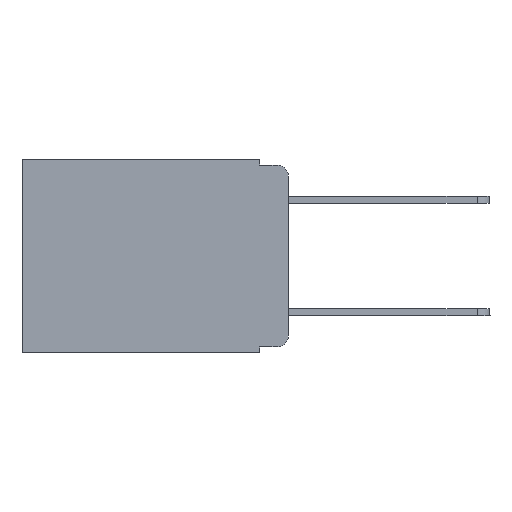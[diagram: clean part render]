
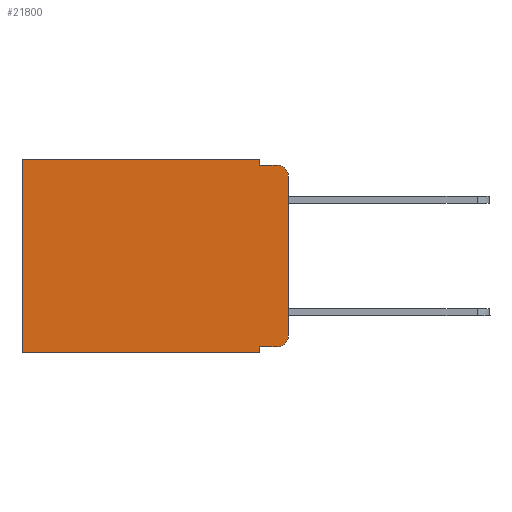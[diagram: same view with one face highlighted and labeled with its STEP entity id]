
A CAD part, left-side view. The second image highlights one B-rep face of the part: STEP entity #21800.
In plain terms, the highlighted planar face has unit normal (-1, 0, 0).
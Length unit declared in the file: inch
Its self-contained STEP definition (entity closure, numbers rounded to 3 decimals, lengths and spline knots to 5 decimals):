
#86 = CARTESIAN_POINT ( 'NONE',  ( 0.298, 0.02, -0.313 ) ) ;
#450 = LINE ( 'NONE', #5903, #1429 ) ;
#1293 = VERTEX_POINT ( 'NONE', #16884 ) ;
#1310 = AXIS2_PLACEMENT_3D ( 'NONE', #14751, #13029, #9602 ) ;
#1429 = VECTOR ( 'NONE', #9416, 39.37008 ) ;
#1767 = ORIENTED_EDGE ( 'NONE', *, *, #3420, .F. ) ;
#1849 = LINE ( 'NONE', #11977, #4859 ) ;
#1903 = LINE ( 'NONE', #16035, #11825 ) ;
#1905 = VERTEX_POINT ( 'NONE', #15480 ) ;
#1956 = LINE ( 'NONE', #10154, #2251 ) ;
#2020 = DIRECTION ( 'NONE',  ( 0., 1., 0. ) ) ;
#2251 = VECTOR ( 'NONE', #13693, 39.37008 ) ;
#2259 = CARTESIAN_POINT ( 'NONE',  ( 0.298, 0., 0. ) ) ;
#2444 = PLANE ( 'NONE',  #1310 ) ;
#2645 = CARTESIAN_POINT ( 'NONE',  ( 0.298, 0., -0.03 ) ) ;
#3133 = DIRECTION ( 'NONE',  ( -1., 0., 0. ) ) ;
#3240 = CARTESIAN_POINT ( 'NONE',  ( 0.298, 0.02, -0.03 ) ) ;
#3420 = EDGE_CURVE ( 'NONE', #14799, #14709, #450, .T. ) ;
#3425 = VECTOR ( 'NONE', #17264, 39.37008 ) ;
#3519 = ORIENTED_EDGE ( 'NONE', *, *, #6052, .F. ) ;
#3616 = DIRECTION ( 'NONE',  ( 0., 0., -1. ) ) ;
#3720 = LINE ( 'NONE', #17625, #22024 ) ;
#3855 = ORIENTED_EDGE ( 'NONE', *, *, #17198, .F. ) ;
#4002 = CARTESIAN_POINT ( 'NONE',  ( 0.298, 0.051, 0. ) ) ;
#4642 = ORIENTED_EDGE ( 'NONE', *, *, #21262, .T. ) ;
#4833 = LINE ( 'NONE', #11771, #11572 ) ;
#4859 = VECTOR ( 'NONE', #8779, 39.37008 ) ;
#4946 = CARTESIAN_POINT ( 'NONE',  ( 0.298, 0.051, -0.01 ) ) ;
#5140 = CIRCLE ( 'NONE', #13151, 0.02 ) ;
#5903 = CARTESIAN_POINT ( 'NONE',  ( 0.298, 0.051, -0.01 ) ) ;
#6052 = EDGE_CURVE ( 'NONE', #12083, #8271, #4833, .T. ) ;
#6919 = DIRECTION ( 'NONE',  ( -1., 0., 0. ) ) ;
#7615 = CARTESIAN_POINT ( 'NONE',  ( 0.298, 0., -0.313 ) ) ;
#8271 = VERTEX_POINT ( 'NONE', #7615 ) ;
#8779 = DIRECTION ( 'NONE',  ( 0., 0., -1. ) ) ;
#8881 = EDGE_CURVE ( 'NONE', #12083, #14709, #5140, .T. ) ;
#9191 = DIRECTION ( 'NONE',  ( 0., 1., 0. ) ) ;
#9244 = VERTEX_POINT ( 'NONE', #14511 ) ;
#9416 = DIRECTION ( 'NONE',  ( 0., -1., 0. ) ) ;
#9452 = EDGE_CURVE ( 'NONE', #16972, #13044, #1956, .T. ) ;
#9602 = DIRECTION ( 'NONE',  ( 0., 0., -1. ) ) ;
#10065 = DIRECTION ( 'NONE',  ( 0., 0., -1. ) ) ;
#10154 = CARTESIAN_POINT ( 'NONE',  ( 0.298, 0.051, -0.333 ) ) ;
#11303 = FACE_OUTER_BOUND ( 'NONE', #18329, .T. ) ;
#11572 = VECTOR ( 'NONE', #18724, 39.37008 ) ;
#11734 = VECTOR ( 'NONE', #9191, 39.37008 ) ;
#11771 = CARTESIAN_POINT ( 'NONE',  ( 0.298, 0., 0. ) ) ;
#11825 = VECTOR ( 'NONE', #3616, 39.37008 ) ;
#11977 = CARTESIAN_POINT ( 'NONE',  ( 0.298, 0.051, 0. ) ) ;
#12024 = CARTESIAN_POINT ( 'NONE',  ( 0.298, 0.051, -0.333 ) ) ;
#12083 = VERTEX_POINT ( 'NONE', #2645 ) ;
#12265 = DIRECTION ( 'NONE',  ( 0., 0., -1. ) ) ;
#12650 = EDGE_CURVE ( 'NONE', #19605, #9244, #17848, .T. ) ;
#13029 = DIRECTION ( 'NONE',  ( 1., 0., 0. ) ) ;
#13044 = VERTEX_POINT ( 'NONE', #16129 ) ;
#13151 = AXIS2_PLACEMENT_3D ( 'NONE', #3240, #3133, #10065 ) ;
#13377 = ORIENTED_EDGE ( 'NONE', *, *, #12650, .T. ) ;
#13693 = DIRECTION ( 'NONE',  ( 0., -1., 0. ) ) ;
#14511 = CARTESIAN_POINT ( 'NONE',  ( 0.298, 0.473, 0. ) ) ;
#14709 = VERTEX_POINT ( 'NONE', #22479 ) ;
#14751 = CARTESIAN_POINT ( 'NONE',  ( 0.298, 0., 0. ) ) ;
#14799 = VERTEX_POINT ( 'NONE', #4946 ) ;
#15480 = CARTESIAN_POINT ( 'NONE',  ( 0.298, 0.051, -0.343 ) ) ;
#16035 = CARTESIAN_POINT ( 'NONE',  ( 0.298, 0.473, 0. ) ) ;
#16129 = CARTESIAN_POINT ( 'NONE',  ( 0.298, 0.02, -0.333 ) ) ;
#16220 = CIRCLE ( 'NONE', #16581, 0.02 ) ;
#16581 = AXIS2_PLACEMENT_3D ( 'NONE', #86, #6919, #12265 ) ;
#16613 = ORIENTED_EDGE ( 'NONE', *, *, #8881, .T. ) ;
#16815 = LINE ( 'NONE', #18735, #3425 ) ;
#16884 = CARTESIAN_POINT ( 'NONE',  ( 0.298, 0.473, -0.343 ) ) ;
#16972 = VERTEX_POINT ( 'NONE', #12024 ) ;
#17148 = EDGE_CURVE ( 'NONE', #13044, #8271, #16220, .T. ) ;
#17198 = EDGE_CURVE ( 'NONE', #1905, #1293, #3720, .T. ) ;
#17264 = DIRECTION ( 'NONE',  ( 0., 0., -1. ) ) ;
#17625 = CARTESIAN_POINT ( 'NONE',  ( 0.298, 0., -0.343 ) ) ;
#17848 = LINE ( 'NONE', #2259, #11734 ) ;
#18057 = ORIENTED_EDGE ( 'NONE', *, *, #17148, .T. ) ;
#18121 = EDGE_CURVE ( 'NONE', #19605, #14799, #1849, .T. ) ;
#18329 = EDGE_LOOP ( 'NONE', ( #3519, #16613, #1767, #20020, #13377, #4642, #3855, #18437, #22100, #18057 ) ) ;
#18437 = ORIENTED_EDGE ( 'NONE', *, *, #18857, .F. ) ;
#18724 = DIRECTION ( 'NONE',  ( 0., 0., -1. ) ) ;
#18735 = CARTESIAN_POINT ( 'NONE',  ( 0.298, 0.051, 0. ) ) ;
#18857 = EDGE_CURVE ( 'NONE', #16972, #1905, #16815, .T. ) ;
#19605 = VERTEX_POINT ( 'NONE', #4002 ) ;
#20020 = ORIENTED_EDGE ( 'NONE', *, *, #18121, .F. ) ;
#21262 = EDGE_CURVE ( 'NONE', #9244, #1293, #1903, .T. ) ;
#21800 = ADVANCED_FACE ( 'NONE', ( #11303 ), #2444, .F. ) ;
#22024 = VECTOR ( 'NONE', #2020, 39.37008 ) ;
#22100 = ORIENTED_EDGE ( 'NONE', *, *, #9452, .T. ) ;
#22479 = CARTESIAN_POINT ( 'NONE',  ( 0.298, 0.02, -0.01 ) ) ;
